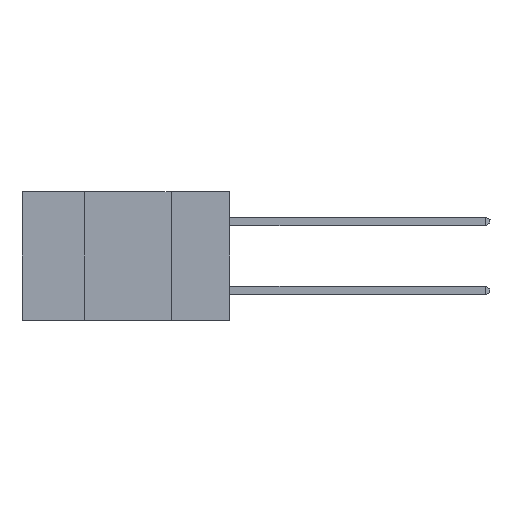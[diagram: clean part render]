
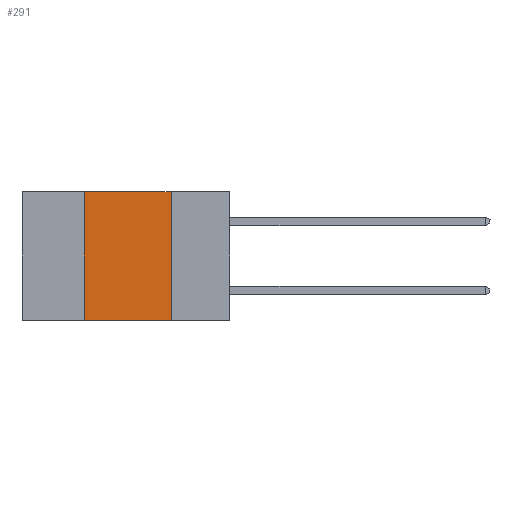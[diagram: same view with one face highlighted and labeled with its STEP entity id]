
A CAD part, left-side view. The second image highlights one B-rep face of the part: STEP entity #291.
In plain terms, the highlighted planar face has unit normal (-1, 0, 0).
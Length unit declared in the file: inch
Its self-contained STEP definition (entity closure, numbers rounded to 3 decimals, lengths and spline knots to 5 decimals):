
#172 = CARTESIAN_POINT ( 'NONE',  ( 0., 0.17, -0.37 ) ) ;
#177 = VERTEX_POINT ( 'NONE', #172 ) ;
#291 = ADVANCED_FACE ( 'NONE', ( #4355 ), #8268, .F. ) ;
#323 = AXIS2_PLACEMENT_3D ( 'NONE', #910, #6627, #5868 ) ;
#416 = EDGE_LOOP ( 'NONE', ( #6220, #1251, #9143, #922 ) ) ;
#910 = CARTESIAN_POINT ( 'NONE',  ( 0., 0.6, 0. ) ) ;
#922 = ORIENTED_EDGE ( 'NONE', *, *, #8048, .T. ) ;
#1251 = ORIENTED_EDGE ( 'NONE', *, *, #9333, .F. ) ;
#1380 = VERTEX_POINT ( 'NONE', #4185 ) ;
#1721 = DIRECTION ( 'NONE',  ( 0., 0., 1. ) ) ;
#1944 = CARTESIAN_POINT ( 'NONE',  ( 0., 0.17, 0. ) ) ;
#3175 = VECTOR ( 'NONE', #1721, 39.37008 ) ;
#4185 = CARTESIAN_POINT ( 'NONE',  ( 0., 0.42, 0. ) ) ;
#4355 = FACE_OUTER_BOUND ( 'NONE', #416, .T. ) ;
#4604 = VERTEX_POINT ( 'NONE', #8275 ) ;
#5395 = CARTESIAN_POINT ( 'NONE',  ( 0., 0.17, 0. ) ) ;
#5517 = EDGE_CURVE ( 'NONE', #4604, #1380, #6901, .T. ) ;
#5651 = EDGE_CURVE ( 'NONE', #10354, #177, #9564, .T. ) ;
#5806 = LINE ( 'NONE', #10519, #6588 ) ;
#5868 = DIRECTION ( 'NONE',  ( 0., 0., -1. ) ) ;
#6220 = ORIENTED_EDGE ( 'NONE', *, *, #5651, .F. ) ;
#6446 = CARTESIAN_POINT ( 'NONE',  ( 0., 0.42, 0. ) ) ;
#6588 = VECTOR ( 'NONE', #8105, 39.37008 ) ;
#6627 = DIRECTION ( 'NONE',  ( 1., 0., 0. ) ) ;
#6901 = LINE ( 'NONE', #6446, #3175 ) ;
#6944 = LINE ( 'NONE', #10420, #7198 ) ;
#7198 = VECTOR ( 'NONE', #10293, 39.37008 ) ;
#7405 = VECTOR ( 'NONE', #9227, 39.37008 ) ;
#8048 = EDGE_CURVE ( 'NONE', #4604, #177, #5806, .T. ) ;
#8105 = DIRECTION ( 'NONE',  ( 0., -1., 0. ) ) ;
#8268 = PLANE ( 'NONE',  #323 ) ;
#8275 = CARTESIAN_POINT ( 'NONE',  ( 0., 0.42, -0.37 ) ) ;
#9143 = ORIENTED_EDGE ( 'NONE', *, *, #5517, .F. ) ;
#9227 = DIRECTION ( 'NONE',  ( 0., 0., -1. ) ) ;
#9333 = EDGE_CURVE ( 'NONE', #1380, #10354, #6944, .T. ) ;
#9564 = LINE ( 'NONE', #1944, #7405 ) ;
#10293 = DIRECTION ( 'NONE',  ( 0., -1., 0. ) ) ;
#10354 = VERTEX_POINT ( 'NONE', #5395 ) ;
#10420 = CARTESIAN_POINT ( 'NONE',  ( 0., 0.6, 0. ) ) ;
#10519 = CARTESIAN_POINT ( 'NONE',  ( 0., 0.6, -0.37 ) ) ;
